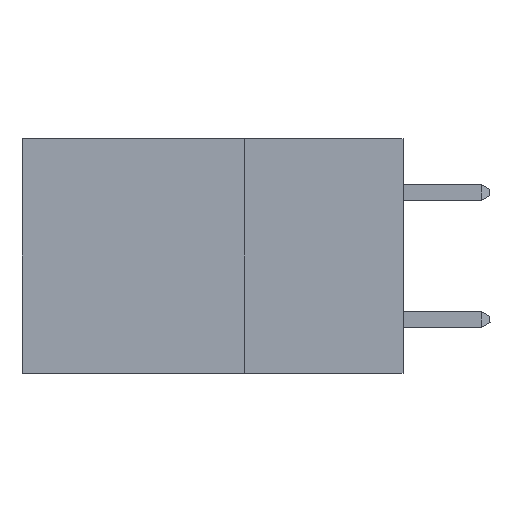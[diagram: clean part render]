
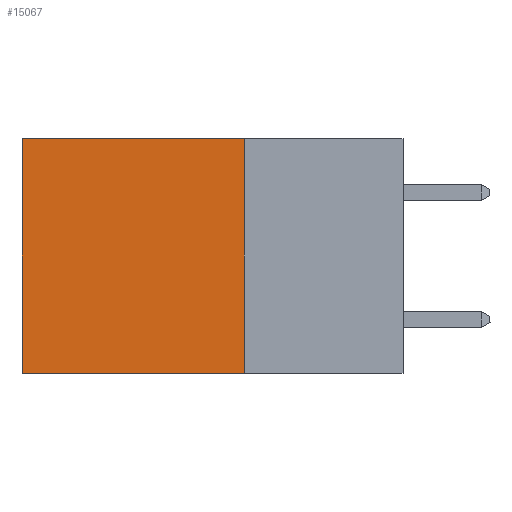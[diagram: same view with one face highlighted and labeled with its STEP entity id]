
A CAD part, left-side view. The second image highlights one B-rep face of the part: STEP entity #15067.
In plain terms, the highlighted planar face has unit normal (-1, 0, 0).
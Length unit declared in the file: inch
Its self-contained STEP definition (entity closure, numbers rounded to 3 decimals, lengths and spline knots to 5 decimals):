
#125 = LINE ( 'NONE', #4084, #1321 ) ;
#228 = LINE ( 'NONE', #11981, #2991 ) ;
#1321 = VECTOR ( 'NONE', #9011, 39.37008 ) ;
#1556 = EDGE_CURVE ( 'NONE', #3195, #10933, #4309, .T. ) ;
#1705 = EDGE_CURVE ( 'NONE', #8763, #10933, #14581, .T. ) ;
#1904 = DIRECTION ( 'NONE',  ( 0., 0., -1. ) ) ;
#2458 = ORIENTED_EDGE ( 'NONE', *, *, #7732, .T. ) ;
#2841 = DIRECTION ( 'NONE',  ( 1., 0., 0. ) ) ;
#2991 = VECTOR ( 'NONE', #5854, 39.37008 ) ;
#3195 = VERTEX_POINT ( 'NONE', #7528 ) ;
#4084 = CARTESIAN_POINT ( 'NONE',  ( 0.2875, 0.25, 0. ) ) ;
#4309 = LINE ( 'NONE', #12863, #8770 ) ;
#5544 = VERTEX_POINT ( 'NONE', #7536 ) ;
#5604 = EDGE_CURVE ( 'NONE', #5544, #3195, #125, .T. ) ;
#5854 = DIRECTION ( 'NONE',  ( 0., 1., 0. ) ) ;
#7445 = ORIENTED_EDGE ( 'NONE', *, *, #5604, .F. ) ;
#7528 = CARTESIAN_POINT ( 'NONE',  ( 0.2875, 0.25, -0.37 ) ) ;
#7536 = CARTESIAN_POINT ( 'NONE',  ( 0.2875, 0.25, 0. ) ) ;
#7732 = EDGE_CURVE ( 'NONE', #5544, #8763, #228, .T. ) ;
#8142 = CARTESIAN_POINT ( 'NONE',  ( 0.2875, 0.6, 0. ) ) ;
#8763 = VERTEX_POINT ( 'NONE', #8142 ) ;
#8770 = VECTOR ( 'NONE', #10499, 39.37008 ) ;
#9011 = DIRECTION ( 'NONE',  ( 0., 0., -1. ) ) ;
#9168 = DIRECTION ( 'NONE',  ( 0., 0., -1. ) ) ;
#9504 = CARTESIAN_POINT ( 'NONE',  ( 0.2875, 0.6, 0. ) ) ;
#9725 = CARTESIAN_POINT ( 'NONE',  ( 0.2875, 0.6, -0.37 ) ) ;
#10350 = FACE_OUTER_BOUND ( 'NONE', #12112, .T. ) ;
#10370 = PLANE ( 'NONE',  #13984 ) ;
#10499 = DIRECTION ( 'NONE',  ( 0., 1., 0. ) ) ;
#10912 = VECTOR ( 'NONE', #1904, 39.37008 ) ;
#10933 = VERTEX_POINT ( 'NONE', #9725 ) ;
#11981 = CARTESIAN_POINT ( 'NONE',  ( 0.2875, 0.25, 0. ) ) ;
#12112 = EDGE_LOOP ( 'NONE', ( #14794, #15004, #7445, #2458 ) ) ;
#12863 = CARTESIAN_POINT ( 'NONE',  ( 0.2875, 0.25, -0.37 ) ) ;
#13868 = CARTESIAN_POINT ( 'NONE',  ( 0.2875, 0.25, 0. ) ) ;
#13984 = AXIS2_PLACEMENT_3D ( 'NONE', #13868, #2841, #9168 ) ;
#14581 = LINE ( 'NONE', #9504, #10912 ) ;
#14794 = ORIENTED_EDGE ( 'NONE', *, *, #1705, .T. ) ;
#15004 = ORIENTED_EDGE ( 'NONE', *, *, #1556, .F. ) ;
#15067 = ADVANCED_FACE ( 'NONE', ( #10350 ), #10370, .F. ) ;
